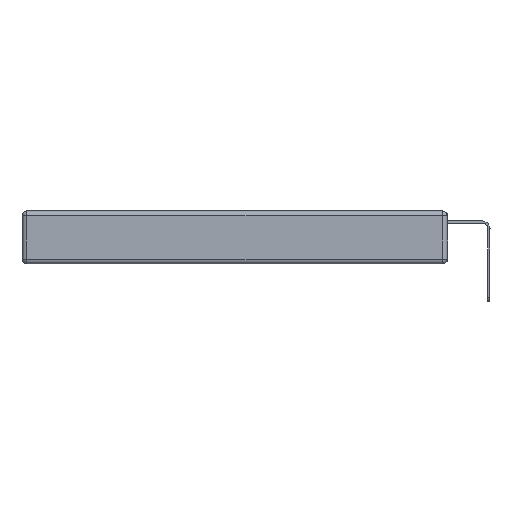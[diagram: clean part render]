
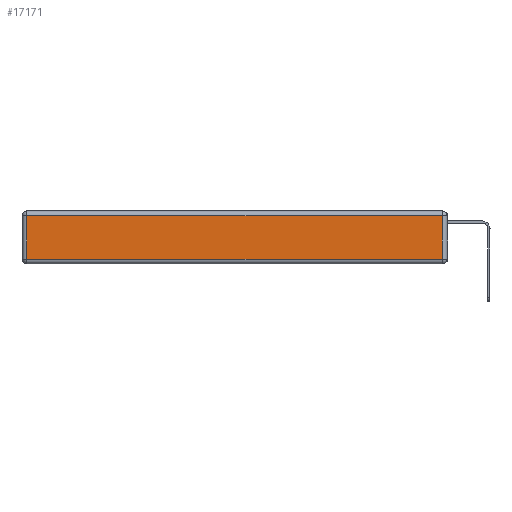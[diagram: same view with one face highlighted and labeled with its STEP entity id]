
A CAD part, left-side view. The second image highlights one B-rep face of the part: STEP entity #17171.
In plain terms, the highlighted planar face has unit normal (-1, 0, 0).
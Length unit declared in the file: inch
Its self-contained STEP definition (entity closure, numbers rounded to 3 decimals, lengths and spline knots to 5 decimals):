
#177 = VECTOR ( 'NONE', #13753, 39.37008 ) ;
#635 = VERTEX_POINT ( 'NONE', #16503 ) ;
#1015 = EDGE_CURVE ( 'NONE', #1769, #16111, #1570, .T. ) ;
#1104 = LINE ( 'NONE', #10817, #14063 ) ;
#1139 = DIRECTION ( 'NONE',  ( 0., 0., 1. ) ) ;
#1570 = LINE ( 'NONE', #9301, #13471 ) ;
#1769 = VERTEX_POINT ( 'NONE', #4560 ) ;
#2527 = CARTESIAN_POINT ( 'NONE',  ( 0., 0., -0.343 ) ) ;
#2550 = AXIS2_PLACEMENT_3D ( 'NONE', #2527, #5472, #6851 ) ;
#2777 = LINE ( 'NONE', #11686, #6163 ) ;
#3521 = EDGE_CURVE ( 'NONE', #635, #1769, #14410, .T. ) ;
#4560 = CARTESIAN_POINT ( 'NONE',  ( 0., 0.03, -0.313 ) ) ;
#4635 = DIRECTION ( 'NONE',  ( 0., 1., 0. ) ) ;
#5367 = ORIENTED_EDGE ( 'NONE', *, *, #3521, .T. ) ;
#5472 = DIRECTION ( 'NONE',  ( -1., 0., 0. ) ) ;
#6163 = VECTOR ( 'NONE', #4635, 39.37008 ) ;
#6851 = DIRECTION ( 'NONE',  ( 0., 0., 1. ) ) ;
#8032 = DIRECTION ( 'NONE',  ( 0., 0., -1. ) ) ;
#9301 = CARTESIAN_POINT ( 'NONE',  ( 0., 0.03, -0.343 ) ) ;
#9527 = VERTEX_POINT ( 'NONE', #9545 ) ;
#9545 = CARTESIAN_POINT ( 'NONE',  ( 0., 2.72, -0.03 ) ) ;
#10817 = CARTESIAN_POINT ( 'NONE',  ( 0., 2.72, -0.343 ) ) ;
#11163 = ORIENTED_EDGE ( 'NONE', *, *, #13179, .T. ) ;
#11686 = CARTESIAN_POINT ( 'NONE',  ( 0., 2.75, -0.03 ) ) ;
#12432 = CARTESIAN_POINT ( 'NONE',  ( 0., 0.03, -0.03 ) ) ;
#13179 = EDGE_CURVE ( 'NONE', #9527, #635, #1104, .T. ) ;
#13372 = PLANE ( 'NONE',  #2550 ) ;
#13471 = VECTOR ( 'NONE', #1139, 39.37008 ) ;
#13576 = CARTESIAN_POINT ( 'NONE',  ( 0., 0., -0.313 ) ) ;
#13617 = EDGE_CURVE ( 'NONE', #16111, #9527, #2777, .T. ) ;
#13753 = DIRECTION ( 'NONE',  ( 0., -1., 0. ) ) ;
#13900 = FACE_OUTER_BOUND ( 'NONE', #16327, .T. ) ;
#14063 = VECTOR ( 'NONE', #8032, 39.37008 ) ;
#14410 = LINE ( 'NONE', #13576, #177 ) ;
#14455 = ORIENTED_EDGE ( 'NONE', *, *, #13617, .T. ) ;
#14579 = ORIENTED_EDGE ( 'NONE', *, *, #1015, .T. ) ;
#16111 = VERTEX_POINT ( 'NONE', #12432 ) ;
#16327 = EDGE_LOOP ( 'NONE', ( #5367, #14579, #14455, #11163 ) ) ;
#16503 = CARTESIAN_POINT ( 'NONE',  ( 0., 2.72, -0.313 ) ) ;
#17171 = ADVANCED_FACE ( 'NONE', ( #13900 ), #13372, .T. ) ;
